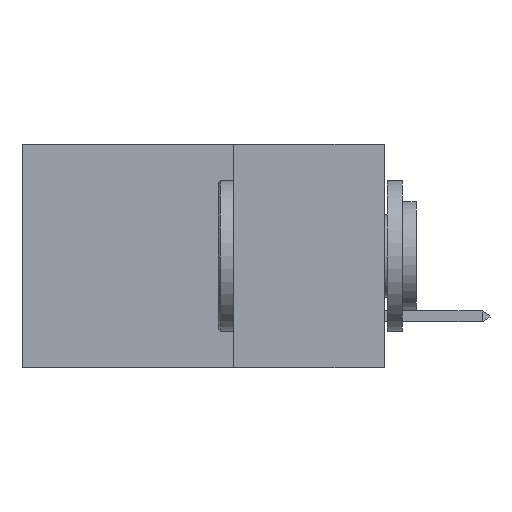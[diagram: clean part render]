
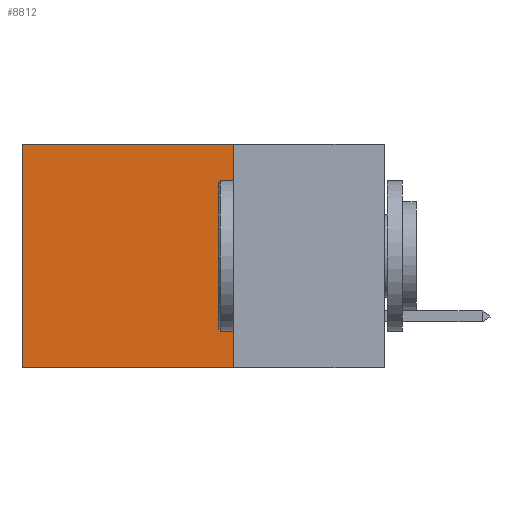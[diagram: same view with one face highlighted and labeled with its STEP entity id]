
A CAD part, left-side view. The second image highlights one B-rep face of the part: STEP entity #8812.
In plain terms, the highlighted planar face has unit normal (-1, 0, 0).
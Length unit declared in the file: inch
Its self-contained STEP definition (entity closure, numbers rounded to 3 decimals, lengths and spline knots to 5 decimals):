
#575 = FACE_OUTER_BOUND ( 'NONE', #25497, .T. ) ;
#1345 = LINE ( 'NONE', #24806, #29734 ) ;
#4348 = VERTEX_POINT ( 'NONE', #21351 ) ;
#6562 = VERTEX_POINT ( 'NONE', #10152 ) ;
#8514 = DIRECTION ( 'NONE',  ( 1., 0., 0. ) ) ;
#8728 = LINE ( 'NONE', #14446, #15181 ) ;
#8812 = ADVANCED_FACE ( 'NONE', ( #575 ), #23076, .F. ) ;
#9314 = EDGE_CURVE ( 'NONE', #27072, #18426, #24241, .T. ) ;
#10152 = CARTESIAN_POINT ( 'NONE',  ( 0.2875, 0.6, -0.37 ) ) ;
#10213 = DIRECTION ( 'NONE',  ( 0., 1., 0. ) ) ;
#10653 = EDGE_CURVE ( 'NONE', #27072, #4348, #15814, .T. ) ;
#12275 = AXIS2_PLACEMENT_3D ( 'NONE', #15733, #8514, #25604 ) ;
#12837 = CARTESIAN_POINT ( 'NONE',  ( 0.2875, 0.25, 0. ) ) ;
#14446 = CARTESIAN_POINT ( 'NONE',  ( 0.2875, 0.6, 0. ) ) ;
#15181 = VECTOR ( 'NONE', #26678, 39.37008 ) ;
#15733 = CARTESIAN_POINT ( 'NONE',  ( 0.2875, 0.25, 0. ) ) ;
#15814 = LINE ( 'NONE', #20305, #23052 ) ;
#18426 = VERTEX_POINT ( 'NONE', #19134 ) ;
#19134 = CARTESIAN_POINT ( 'NONE',  ( 0.2875, 0.6, 0. ) ) ;
#20305 = CARTESIAN_POINT ( 'NONE',  ( 0.2875, 0.25, 0. ) ) ;
#21351 = CARTESIAN_POINT ( 'NONE',  ( 0.2875, 0.25, -0.37 ) ) ;
#22268 = EDGE_CURVE ( 'NONE', #4348, #6562, #1345, .T. ) ;
#22436 = ORIENTED_EDGE ( 'NONE', *, *, #9314, .T. ) ;
#23052 = VECTOR ( 'NONE', #30162, 39.37008 ) ;
#23076 = PLANE ( 'NONE',  #12275 ) ;
#24241 = LINE ( 'NONE', #12837, #25831 ) ;
#24653 = ORIENTED_EDGE ( 'NONE', *, *, #27482, .T. ) ;
#24806 = CARTESIAN_POINT ( 'NONE',  ( 0.2875, 0.25, -0.37 ) ) ;
#25497 = EDGE_LOOP ( 'NONE', ( #24653, #30934, #26543, #22436 ) ) ;
#25604 = DIRECTION ( 'NONE',  ( 0., 0., -1. ) ) ;
#25831 = VECTOR ( 'NONE', #27522, 39.37008 ) ;
#26543 = ORIENTED_EDGE ( 'NONE', *, *, #10653, .F. ) ;
#26678 = DIRECTION ( 'NONE',  ( 0., 0., -1. ) ) ;
#27072 = VERTEX_POINT ( 'NONE', #27665 ) ;
#27482 = EDGE_CURVE ( 'NONE', #18426, #6562, #8728, .T. ) ;
#27522 = DIRECTION ( 'NONE',  ( 0., 1., 0. ) ) ;
#27665 = CARTESIAN_POINT ( 'NONE',  ( 0.2875, 0.25, 0. ) ) ;
#29734 = VECTOR ( 'NONE', #10213, 39.37008 ) ;
#30162 = DIRECTION ( 'NONE',  ( 0., 0., -1. ) ) ;
#30934 = ORIENTED_EDGE ( 'NONE', *, *, #22268, .F. ) ;
